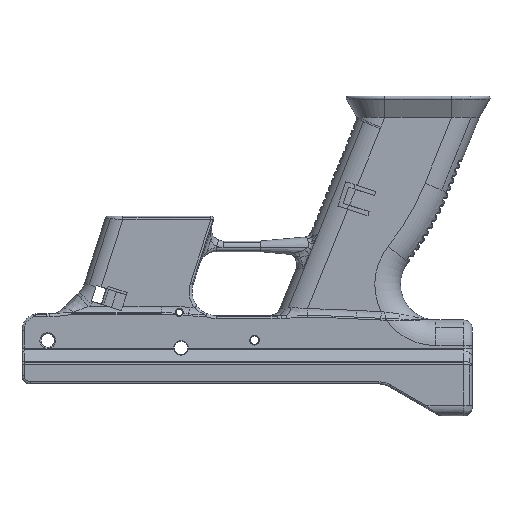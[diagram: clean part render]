
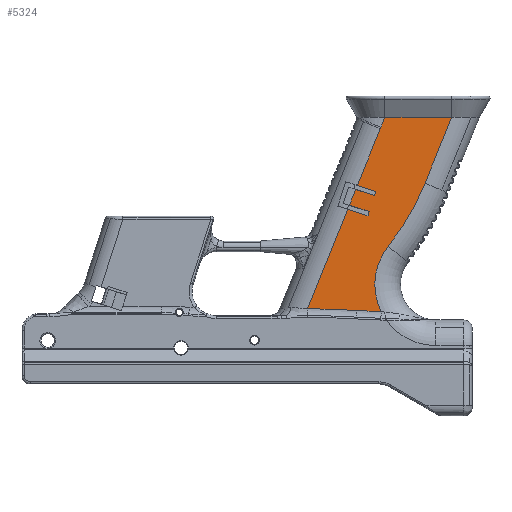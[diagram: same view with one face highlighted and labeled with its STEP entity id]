
A CAD part, front view. The second image highlights one B-rep face of the part: STEP entity #5324.
In plain terms, the highlighted planar face has unit normal (0, -1, 0).
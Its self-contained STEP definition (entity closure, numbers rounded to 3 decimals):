
#243 = EDGE_CURVE ( 'NONE', #18464, #40572, #32241, .T. ) ;
#305 = DIRECTION ( 'NONE',  ( 0.375, 0., 0.927 ) ) ;
#818 = EDGE_LOOP ( 'NONE', ( #51659, #18326, #36761, #30038, #9256, #31258, #9310, #29909, #14292, #25366, #7176, #17210, #48598, #34202, #36640, #51269, #20077 ) ) ;
#971 = CARTESIAN_POINT ( 'NONE',  ( 72.175, -14.625, 29.078 ) ) ;
#1351 = LINE ( 'NONE', #34010, #26781 ) ;
#1499 = LINE ( 'NONE', #2039, #43023 ) ;
#1685 = VERTEX_POINT ( 'NONE', #50773 ) ;
#1729 = CARTESIAN_POINT ( 'NONE',  ( 53.832, -14.625, -61.703 ) ) ;
#2039 = CARTESIAN_POINT ( 'NONE',  ( 88.836, -14.625, -7.677 ) ) ;
#2648 = EDGE_CURVE ( 'NONE', #3205, #27212, #32598, .T. ) ;
#2904 = DIRECTION ( 'NONE',  ( 0.375, 0., 0.927 ) ) ;
#3166 = CARTESIAN_POINT ( 'NONE',  ( 90.04, -14.625, 27.958 ) ) ;
#3205 = VERTEX_POINT ( 'NONE', #30369 ) ;
#3442 = VECTOR ( 'NONE', #2904, 1000. ) ;
#4466 = AXIS2_PLACEMENT_3D ( 'NONE', #5458, #34331, #42142 ) ;
#4723 = CARTESIAN_POINT ( 'NONE',  ( 39.557, -14.625, -757.86 ) ) ;
#5324 = ADVANCED_FACE ( 'NONE', ( #33983 ), #49797, .T. ) ;
#5458 = CARTESIAN_POINT ( 'NONE',  ( -1.344, -14.625, 41.627 ) ) ;
#5473 = CARTESIAN_POINT ( 'NONE',  ( 121.365, -14.625, 27.958 ) ) ;
#6813 = EDGE_CURVE ( 'NONE', #9958, #49143, #23165, .T. ) ;
#6829 = CARTESIAN_POINT ( 'NONE',  ( 2.375, -14.625, 7.416 ) ) ;
#7169 = VECTOR ( 'NONE', #24858, 1000. ) ;
#7176 = ORIENTED_EDGE ( 'NONE', *, *, #6813, .T. ) ;
#7522 = AXIS2_PLACEMENT_3D ( 'NONE', #971, #41461, #45716 ) ;
#8106 = LINE ( 'NONE', #28973, #19874 ) ;
#9194 = EDGE_CURVE ( 'NONE', #27212, #49143, #19484, .T. ) ;
#9256 = ORIENTED_EDGE ( 'NONE', *, *, #243, .F. ) ;
#9296 = DIRECTION ( 'NONE',  ( 0., 1., 0. ) ) ;
#9310 = ORIENTED_EDGE ( 'NONE', *, *, #33466, .F. ) ;
#9958 = VERTEX_POINT ( 'NONE', #3166 ) ;
#11328 = VERTEX_POINT ( 'NONE', #38521 ) ;
#11515 = EDGE_CURVE ( 'NONE', #50981, #11328, #33867, .T. ) ;
#12485 = DIRECTION ( 'NONE',  ( -0.054, 0., -0.999 ) ) ;
#12564 = LINE ( 'NONE', #17352, #7169 ) ;
#12614 = DIRECTION ( 'NONE',  ( 0., 0., -1. ) ) ;
#12753 = CARTESIAN_POINT ( 'NONE',  ( 87.937, -14.625, 22.71 ) ) ;
#12951 = VECTOR ( 'NONE', #31798, 1000. ) ;
#14089 = VERTEX_POINT ( 'NONE', #23012 ) ;
#14292 = ORIENTED_EDGE ( 'NONE', *, *, #11515, .F. ) ;
#14449 = VERTEX_POINT ( 'NONE', #39545 ) ;
#14904 = CARTESIAN_POINT ( 'NONE',  ( 76.418, -14.625, -5.799 ) ) ;
#16191 = DIRECTION ( 'NONE',  ( -0.375, 0., -0.927 ) ) ;
#16365 = CARTESIAN_POINT ( 'NONE',  ( 70.22, -14.625, -21.141 ) ) ;
#16874 = EDGE_CURVE ( 'NONE', #3205, #29763, #1499, .T. ) ;
#16983 = EDGE_CURVE ( 'NONE', #14449, #18464, #32786, .T. ) ;
#17210 = ORIENTED_EDGE ( 'NONE', *, *, #9194, .F. ) ;
#17352 = CARTESIAN_POINT ( 'NONE',  ( 69.665, -14.625, 27.958 ) ) ;
#18016 = CARTESIAN_POINT ( 'NONE',  ( 113.981, -14.625, -50.37 ) ) ;
#18326 = ORIENTED_EDGE ( 'NONE', *, *, #51428, .T. ) ;
#18464 = VERTEX_POINT ( 'NONE', #33872 ) ;
#18617 = DIRECTION ( 'NONE',  ( -0.952, 0., 0.305 ) ) ;
#18838 = VECTOR ( 'NONE', #33896, 1000. ) ;
#19484 = CIRCLE ( 'NONE', #7522, 17. ) ;
#19874 = VECTOR ( 'NONE', #24442, 1000. ) ;
#20077 = ORIENTED_EDGE ( 'NONE', *, *, #20676, .F. ) ;
#20674 = VECTOR ( 'NONE', #18617, 1000. ) ;
#20676 = EDGE_CURVE ( 'NONE', #1685, #26970, #1351, .T. ) ;
#21324 = EDGE_CURVE ( 'NONE', #11328, #37931, #45513, .T. ) ;
#21394 = EDGE_CURVE ( 'NONE', #29763, #14089, #8106, .T. ) ;
#21524 = DIRECTION ( 'NONE',  ( 0.782, 0., -0.624 ) ) ;
#22008 = AXIS2_PLACEMENT_3D ( 'NONE', #4723, #45670, #12485 ) ;
#23012 = CARTESIAN_POINT ( 'NONE',  ( 85.222, -14.625, -8.619 ) ) ;
#23165 = LINE ( 'NONE', #39498, #48940 ) ;
#23347 = AXIS2_PLACEMENT_3D ( 'NONE', #45973, #9296, #25629 ) ;
#23595 = VERTEX_POINT ( 'NONE', #35619 ) ;
#24066 = VECTOR ( 'NONE', #305, 1000. ) ;
#24442 = DIRECTION ( 'NONE',  ( -0.305, 0., -0.952 ) ) ;
#24858 = DIRECTION ( 'NONE',  ( 1., 0., 0. ) ) ;
#25223 = CARTESIAN_POINT ( 'NONE',  ( 88.199, -14.625, 23.402 ) ) ;
#25366 = ORIENTED_EDGE ( 'NONE', *, *, #26832, .F. ) ;
#25629 = DIRECTION ( 'NONE',  ( 0.037, 0., 0.999 ) ) ;
#26307 = CARTESIAN_POINT ( 'NONE',  ( 91.6, -14.625, -32.517 ) ) ;
#26721 = VECTOR ( 'NONE', #36166, 1000. ) ;
#26781 = VECTOR ( 'NONE', #37261, 1000. ) ;
#26832 = EDGE_CURVE ( 'NONE', #9958, #50981, #12564, .T. ) ;
#26970 = VERTEX_POINT ( 'NONE', #14904 ) ;
#27212 = VERTEX_POINT ( 'NONE', #12753 ) ;
#27331 = CARTESIAN_POINT ( 'NONE',  ( 88.226, -14.625, -9.581 ) ) ;
#27860 = CARTESIAN_POINT ( 'NONE',  ( 82.172, -14.625, -18.143 ) ) ;
#28973 = CARTESIAN_POINT ( 'NONE',  ( 79.797, -14.625, -25.559 ) ) ;
#29566 = DIRECTION ( 'NONE',  ( 0., -1., 0. ) ) ;
#29763 = VERTEX_POINT ( 'NONE', #32813 ) ;
#29909 = ORIENTED_EDGE ( 'NONE', *, *, #21324, .F. ) ;
#29965 = DIRECTION ( 'NONE',  ( 0., -1., 0. ) ) ;
#30038 = ORIENTED_EDGE ( 'NONE', *, *, #31809, .F. ) ;
#30369 = CARTESIAN_POINT ( 'NONE',  ( 77.169, -14.625, -3.94 ) ) ;
#31037 = AXIS2_PLACEMENT_3D ( 'NONE', #37741, #29965, #12614 ) ;
#31258 = ORIENTED_EDGE ( 'NONE', *, *, #16983, .F. ) ;
#31412 = EDGE_CURVE ( 'NONE', #26970, #14089, #35883, .T. ) ;
#31798 = DIRECTION ( 'NONE',  ( -0.305, 0., -0.952 ) ) ;
#31809 = EDGE_CURVE ( 'NONE', #40572, #23595, #36710, .T. ) ;
#32241 = CIRCLE ( 'NONE', #22008, 696.304 ) ;
#32598 = LINE ( 'NONE', #35817, #3442 ) ;
#32786 = CIRCLE ( 'NONE', #23347, 689.416 ) ;
#32813 = CARTESIAN_POINT ( 'NONE',  ( 85.832, -14.625, -6.715 ) ) ;
#33401 = EDGE_CURVE ( 'NONE', #50017, #23595, #43500, .T. ) ;
#33466 = EDGE_CURVE ( 'NONE', #37931, #14449, #42897, .T. ) ;
#33867 = LINE ( 'NONE', #37886, #50012 ) ;
#33872 = CARTESIAN_POINT ( 'NONE',  ( 76.954, -14.625, -62.561 ) ) ;
#33896 = DIRECTION ( 'NONE',  ( -0.952, 0., 0.305 ) ) ;
#33983 = FACE_OUTER_BOUND ( 'NONE', #818, .T. ) ;
#34010 = CARTESIAN_POINT ( 'NONE',  ( 70.22, -14.625, -21.141 ) ) ;
#34147 = CARTESIAN_POINT ( 'NONE',  ( 2.985, -14.625, 9.32 ) ) ;
#34202 = ORIENTED_EDGE ( 'NONE', *, *, #16874, .T. ) ;
#34331 = DIRECTION ( 'NONE',  ( 0., 1., 0. ) ) ;
#35619 = CARTESIAN_POINT ( 'NONE',  ( 72.662, -14.625, -15.097 ) ) ;
#35817 = CARTESIAN_POINT ( 'NONE',  ( 70.22, -14.625, -21.141 ) ) ;
#35883 = LINE ( 'NONE', #27331, #26721 ) ;
#36166 = DIRECTION ( 'NONE',  ( 0.952, 0., -0.305 ) ) ;
#36640 = ORIENTED_EDGE ( 'NONE', *, *, #21394, .T. ) ;
#36710 = LINE ( 'NONE', #16365, #24066 ) ;
#36761 = ORIENTED_EDGE ( 'NONE', *, *, #33401, .T. ) ;
#37261 = DIRECTION ( 'NONE',  ( 0.375, 0., 0.927 ) ) ;
#37741 = CARTESIAN_POINT ( 'NONE',  ( 86.464, -14.625, -15.081 ) ) ;
#37886 = CARTESIAN_POINT ( 'NONE',  ( 111.761, -14.625, 4.188 ) ) ;
#37931 = VERTEX_POINT ( 'NONE', #26307 ) ;
#38006 = VERTEX_POINT ( 'NONE', #47158 ) ;
#38521 = CARTESIAN_POINT ( 'NONE',  ( 108.893, -14.625, -2.912 ) ) ;
#39498 = CARTESIAN_POINT ( 'NONE',  ( 106.929, -14.625, 69.761 ) ) ;
#39545 = CARTESIAN_POINT ( 'NONE',  ( 88.326, -14.625, -63.079 ) ) ;
#40572 = VERTEX_POINT ( 'NONE', #1729 ) ;
#40680 = DIRECTION ( 'NONE',  ( -0.375, 0., -0.927 ) ) ;
#41461 = DIRECTION ( 'NONE',  ( 0., -1., 0. ) ) ;
#42078 = AXIS2_PLACEMENT_3D ( 'NONE', #18016, #29566, #21524 ) ;
#42142 = DIRECTION ( 'NONE',  ( 0.891, 0., -0.454 ) ) ;
#42486 = DIRECTION ( 'NONE',  ( 0.952, 0., -0.305 ) ) ;
#42897 = CIRCLE ( 'NONE', #42078, 28.63 ) ;
#43023 = VECTOR ( 'NONE', #42486, 1000. ) ;
#43500 = LINE ( 'NONE', #6829, #20674 ) ;
#44395 = LINE ( 'NONE', #47605, #12951 ) ;
#45513 = CIRCLE ( 'NONE', #4466, 118.894 ) ;
#45670 = DIRECTION ( 'NONE',  ( 0., -1., 0. ) ) ;
#45699 = LINE ( 'NONE', #34147, #18838 ) ;
#45716 = DIRECTION ( 'NONE',  ( 0.992, 0., 0.126 ) ) ;
#45752 = EDGE_CURVE ( 'NONE', #38006, #1685, #45699, .T. ) ;
#45973 = CARTESIAN_POINT ( 'NONE',  ( 113.981, -14.625, 625.86 ) ) ;
#47158 = CARTESIAN_POINT ( 'NONE',  ( 82.782, -14.625, -16.238 ) ) ;
#47605 = CARTESIAN_POINT ( 'NONE',  ( 79.797, -14.625, -25.559 ) ) ;
#48598 = ORIENTED_EDGE ( 'NONE', *, *, #2648, .F. ) ;
#48940 = VECTOR ( 'NONE', #16191, 1000. ) ;
#49143 = VERTEX_POINT ( 'NONE', #25223 ) ;
#49797 = PLANE ( 'NONE',  #31037 ) ;
#50012 = VECTOR ( 'NONE', #40680, 1000. ) ;
#50017 = VERTEX_POINT ( 'NONE', #27860 ) ;
#50773 = CARTESIAN_POINT ( 'NONE',  ( 73.413, -14.625, -13.237 ) ) ;
#50981 = VERTEX_POINT ( 'NONE', #5473 ) ;
#51269 = ORIENTED_EDGE ( 'NONE', *, *, #31412, .F. ) ;
#51428 = EDGE_CURVE ( 'NONE', #38006, #50017, #44395, .T. ) ;
#51659 = ORIENTED_EDGE ( 'NONE', *, *, #45752, .F. ) ;
